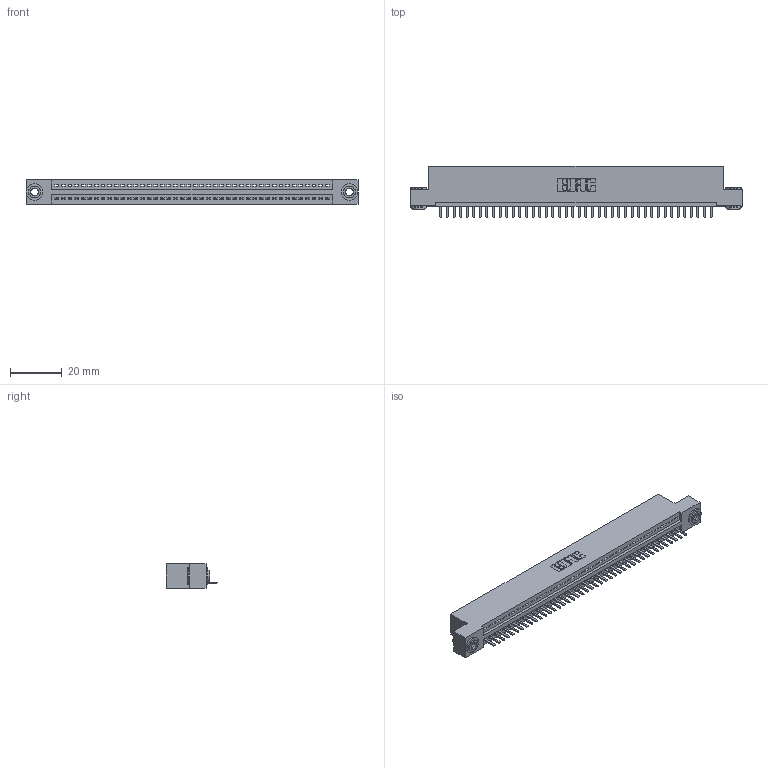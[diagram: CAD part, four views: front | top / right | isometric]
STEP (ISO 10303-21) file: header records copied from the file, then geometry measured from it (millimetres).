
FILE_DESCRIPTION (( 'STEP AP203' ), '1' );
FILE_NAME ('395-042-520-103.STEP', '2019-10-22T11:29:43', ( '' ), ( '' ), 'SwSTEP 2.0', 'SolidWorks 2016', '' );
FILE_SCHEMA (( 'CONFIG_CONTROL_DESIGN' ));
Length unit declared in the file: inch
Products named in the file (4): 345 Part_Flush Mounting Lugs - 0.156 Dia-TH; 345-250-002_345-250-002-102; 395-042-520-103; 345-292-001_345-293-120
Assembly tree (45 placements, depth 2):
  395-042-520-103
    345 Part_Flush Mounting Lugs - 0.156 Dia-TH
    345-292-001_345-293-120  x42
    345-250-002_345-250-002-102  x2
Bounding box: 127.89 x 19.68 x 9.4 mm (x, y, z)
Volume: 12045.6 mm3; surface area: 15826.8 mm2
Topology: 45 solids, 45 shells, 2768 faces, 8145 edges, 5314 vertices
Faces by surface type: plane 1854, cylinder 906, cone 8
Entity records: 32374 total; most frequent: CARTESIAN_POINT 5597, ORIENTED_EDGE 5554, DIRECTION 4907, EDGE_CURVE 2777, VECTOR 2449, LINE 2449, VERTEX_POINT 1846, AXIS2_PLACEMENT_3D 1229
